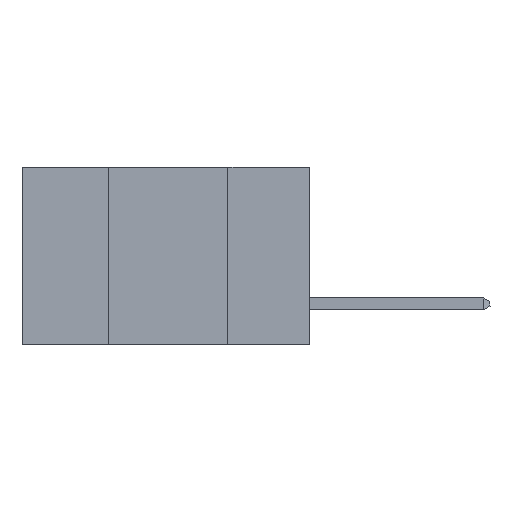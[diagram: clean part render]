
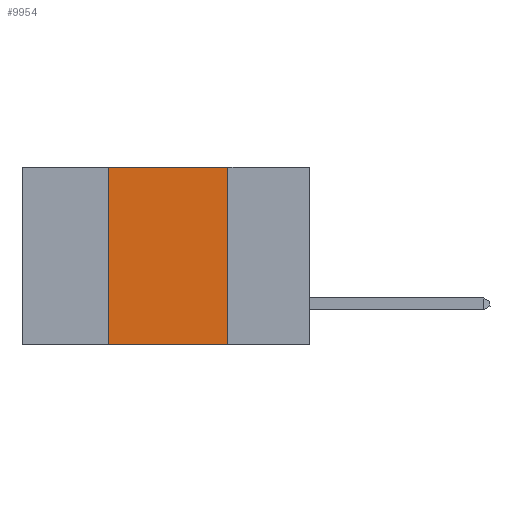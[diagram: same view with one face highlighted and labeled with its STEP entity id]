
A CAD part, left-side view. The second image highlights one B-rep face of the part: STEP entity #9954.
In plain terms, the highlighted planar face has unit normal (-1, 0, 0).
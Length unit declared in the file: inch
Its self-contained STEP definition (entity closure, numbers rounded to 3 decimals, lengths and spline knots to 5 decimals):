
#758 = VECTOR ( 'NONE', #12521, 39.37008 ) ;
#1760 = PLANE ( 'NONE',  #18075 ) ;
#2480 = FACE_OUTER_BOUND ( 'NONE', #12199, .T. ) ;
#3592 = DIRECTION ( 'NONE',  ( 1., 0., 0. ) ) ;
#4312 = CARTESIAN_POINT ( 'NONE',  ( 0., 0.6, 0. ) ) ;
#4843 = LINE ( 'NONE', #5830, #13088 ) ;
#5291 = EDGE_CURVE ( 'NONE', #9135, #14576, #15865, .T. ) ;
#5830 = CARTESIAN_POINT ( 'NONE',  ( 0., 0.6, -0.37 ) ) ;
#7578 = DIRECTION ( 'NONE',  ( 0., -1., 0. ) ) ;
#7690 = ORIENTED_EDGE ( 'NONE', *, *, #19132, .F. ) ;
#8792 = ORIENTED_EDGE ( 'NONE', *, *, #15830, .T. ) ;
#9135 = VERTEX_POINT ( 'NONE', #13341 ) ;
#9954 = ADVANCED_FACE ( 'NONE', ( #2480 ), #1760, .F. ) ;
#10008 = EDGE_CURVE ( 'NONE', #14712, #15568, #19384, .T. ) ;
#11528 = CARTESIAN_POINT ( 'NONE',  ( 0., 0.42, -0.37 ) ) ;
#12199 = EDGE_LOOP ( 'NONE', ( #16429, #7690, #17501, #8792 ) ) ;
#12521 = DIRECTION ( 'NONE',  ( 0., 0., 1. ) ) ;
#13088 = VECTOR ( 'NONE', #7578, 39.37008 ) ;
#13341 = CARTESIAN_POINT ( 'NONE',  ( 0., 0.17, 0. ) ) ;
#13452 = CARTESIAN_POINT ( 'NONE',  ( 0., 0.17, 0. ) ) ;
#14128 = CARTESIAN_POINT ( 'NONE',  ( 0., 0.6, 0. ) ) ;
#14576 = VERTEX_POINT ( 'NONE', #19704 ) ;
#14712 = VERTEX_POINT ( 'NONE', #11528 ) ;
#15568 = VERTEX_POINT ( 'NONE', #20641 ) ;
#15830 = EDGE_CURVE ( 'NONE', #14712, #14576, #4843, .T. ) ;
#15861 = DIRECTION ( 'NONE',  ( 0., 0., -1. ) ) ;
#15865 = LINE ( 'NONE', #13452, #20307 ) ;
#16429 = ORIENTED_EDGE ( 'NONE', *, *, #5291, .F. ) ;
#17501 = ORIENTED_EDGE ( 'NONE', *, *, #10008, .F. ) ;
#18075 = AXIS2_PLACEMENT_3D ( 'NONE', #14128, #3592, #15861 ) ;
#18608 = DIRECTION ( 'NONE',  ( 0., 0., -1. ) ) ;
#19132 = EDGE_CURVE ( 'NONE', #15568, #9135, #21050, .T. ) ;
#19384 = LINE ( 'NONE', #20966, #758 ) ;
#19704 = CARTESIAN_POINT ( 'NONE',  ( 0., 0.17, -0.37 ) ) ;
#20307 = VECTOR ( 'NONE', #18608, 39.37008 ) ;
#20532 = VECTOR ( 'NONE', #21543, 39.37008 ) ;
#20641 = CARTESIAN_POINT ( 'NONE',  ( 0., 0.42, 0. ) ) ;
#20966 = CARTESIAN_POINT ( 'NONE',  ( 0., 0.42, 0. ) ) ;
#21050 = LINE ( 'NONE', #4312, #20532 ) ;
#21543 = DIRECTION ( 'NONE',  ( 0., -1., 0. ) ) ;
